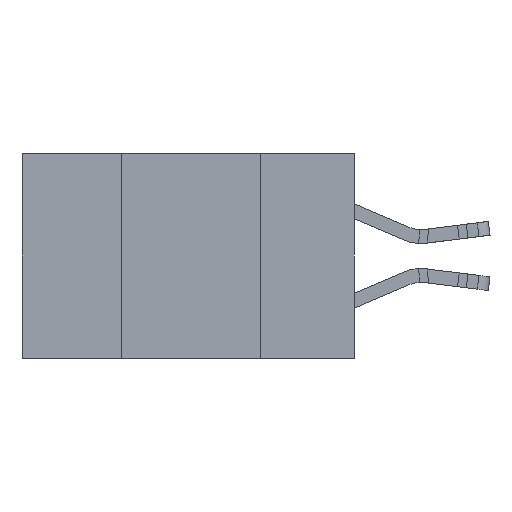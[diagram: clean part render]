
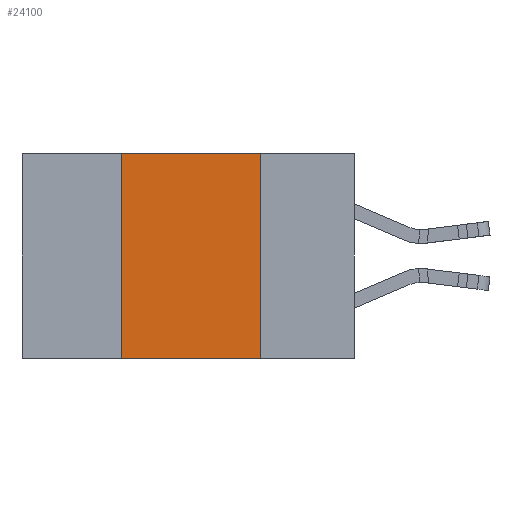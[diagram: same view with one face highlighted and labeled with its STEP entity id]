
A CAD part, left-side view. The second image highlights one B-rep face of the part: STEP entity #24100.
In plain terms, the highlighted planar face has unit normal (-1, 0, 0).
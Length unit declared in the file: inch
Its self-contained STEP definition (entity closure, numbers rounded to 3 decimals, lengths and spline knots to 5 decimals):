
#188 = VERTEX_POINT ( 'NONE', #13609 ) ;
#307 = VECTOR ( 'NONE', #12201, 39.37008 ) ;
#687 = VECTOR ( 'NONE', #22146, 39.37008 ) ;
#992 = CARTESIAN_POINT ( 'NONE',  ( 0., 0.6, 0. ) ) ;
#4920 = EDGE_CURVE ( 'NONE', #188, #11654, #7020, .T. ) ;
#6294 = CARTESIAN_POINT ( 'NONE',  ( 0., 0.6, 0. ) ) ;
#7020 = LINE ( 'NONE', #15397, #16190 ) ;
#7156 = DIRECTION ( 'NONE',  ( 0., -1., 0. ) ) ;
#7331 = AXIS2_PLACEMENT_3D ( 'NONE', #6294, #21567, #23044 ) ;
#8694 = VERTEX_POINT ( 'NONE', #24284 ) ;
#11654 = VERTEX_POINT ( 'NONE', #21144 ) ;
#11684 = LINE ( 'NONE', #27073, #307 ) ;
#12173 = EDGE_LOOP ( 'NONE', ( #15203, #23453, #20593, #21609 ) ) ;
#12201 = DIRECTION ( 'NONE',  ( 0., 0., -1. ) ) ;
#13609 = CARTESIAN_POINT ( 'NONE',  ( 0., 0.42, -0.37 ) ) ;
#14083 = VERTEX_POINT ( 'NONE', #17902 ) ;
#15203 = ORIENTED_EDGE ( 'NONE', *, *, #23504, .F. ) ;
#15397 = CARTESIAN_POINT ( 'NONE',  ( 0., 0.6, -0.37 ) ) ;
#15539 = LINE ( 'NONE', #992, #687 ) ;
#16190 = VECTOR ( 'NONE', #7156, 39.37008 ) ;
#16258 = EDGE_CURVE ( 'NONE', #188, #8694, #19005, .T. ) ;
#16430 = VECTOR ( 'NONE', #23521, 39.37008 ) ;
#16512 = EDGE_CURVE ( 'NONE', #8694, #14083, #15539, .T. ) ;
#17902 = CARTESIAN_POINT ( 'NONE',  ( 0., 0.17, 0. ) ) ;
#19005 = LINE ( 'NONE', #25623, #16430 ) ;
#19214 = FACE_OUTER_BOUND ( 'NONE', #12173, .T. ) ;
#20593 = ORIENTED_EDGE ( 'NONE', *, *, #16258, .F. ) ;
#21144 = CARTESIAN_POINT ( 'NONE',  ( 0., 0.17, -0.37 ) ) ;
#21567 = DIRECTION ( 'NONE',  ( 1., 0., 0. ) ) ;
#21609 = ORIENTED_EDGE ( 'NONE', *, *, #4920, .T. ) ;
#22146 = DIRECTION ( 'NONE',  ( 0., -1., 0. ) ) ;
#23044 = DIRECTION ( 'NONE',  ( 0., 0., -1. ) ) ;
#23453 = ORIENTED_EDGE ( 'NONE', *, *, #16512, .F. ) ;
#23504 = EDGE_CURVE ( 'NONE', #14083, #11654, #11684, .T. ) ;
#23521 = DIRECTION ( 'NONE',  ( 0., 0., 1. ) ) ;
#24100 = ADVANCED_FACE ( 'NONE', ( #19214 ), #25558, .F. ) ;
#24284 = CARTESIAN_POINT ( 'NONE',  ( 0., 0.42, 0. ) ) ;
#25558 = PLANE ( 'NONE',  #7331 ) ;
#25623 = CARTESIAN_POINT ( 'NONE',  ( 0., 0.42, -0.37 ) ) ;
#27073 = CARTESIAN_POINT ( 'NONE',  ( 0., 0.17, -0.37 ) ) ;
